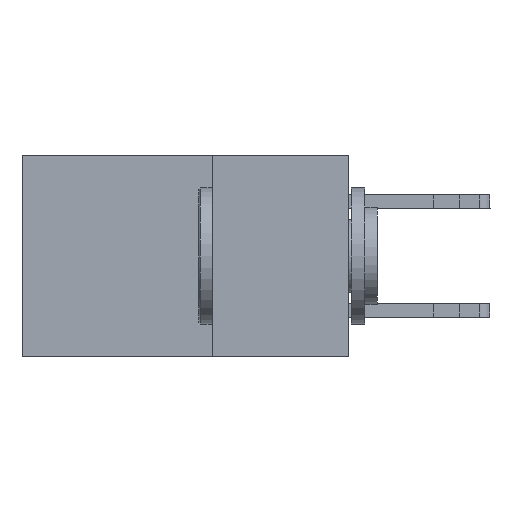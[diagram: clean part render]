
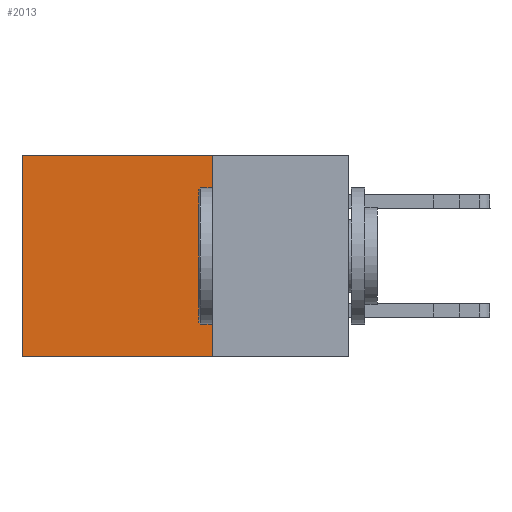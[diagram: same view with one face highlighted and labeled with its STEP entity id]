
A CAD part, left-side view. The second image highlights one B-rep face of the part: STEP entity #2013.
In plain terms, the highlighted planar face has unit normal (-1, 0, 0).
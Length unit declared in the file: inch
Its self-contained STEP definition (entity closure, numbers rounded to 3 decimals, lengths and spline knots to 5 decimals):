
#376 = CARTESIAN_POINT ( 'NONE',  ( 0.2615, 0.25, -0.37 ) ) ;
#753 = EDGE_LOOP ( 'NONE', ( #884, #5151, #13641, #5971 ) ) ;
#847 = CARTESIAN_POINT ( 'NONE',  ( 0.2615, 0.6, -0.37 ) ) ;
#884 = ORIENTED_EDGE ( 'NONE', *, *, #1803, .T. ) ;
#984 = CARTESIAN_POINT ( 'NONE',  ( 0.2615, 0.25, -0.37 ) ) ;
#1065 = FACE_OUTER_BOUND ( 'NONE', #753, .T. ) ;
#1489 = CARTESIAN_POINT ( 'NONE',  ( 0.2615, 0.6, 0. ) ) ;
#1803 = EDGE_CURVE ( 'NONE', #11280, #7477, #9476, .T. ) ;
#2013 = ADVANCED_FACE ( 'NONE', ( #1065 ), #5429, .F. ) ;
#2033 = EDGE_CURVE ( 'NONE', #10538, #4197, #12306, .T. ) ;
#2345 = CARTESIAN_POINT ( 'NONE',  ( 0.2615, 0.25, -0.37 ) ) ;
#3727 = EDGE_CURVE ( 'NONE', #4197, #7477, #8338, .T. ) ;
#4197 = VERTEX_POINT ( 'NONE', #376 ) ;
#4408 = CARTESIAN_POINT ( 'NONE',  ( 0.2615, 0.25, 0. ) ) ;
#5151 = ORIENTED_EDGE ( 'NONE', *, *, #3727, .F. ) ;
#5202 = DIRECTION ( 'NONE',  ( 0., 1., 0. ) ) ;
#5429 = PLANE ( 'NONE',  #5940 ) ;
#5575 = DIRECTION ( 'NONE',  ( 1., 0., 0. ) ) ;
#5940 = AXIS2_PLACEMENT_3D ( 'NONE', #984, #5575, #10065 ) ;
#5971 = ORIENTED_EDGE ( 'NONE', *, *, #13372, .T. ) ;
#6360 = VECTOR ( 'NONE', #7772, 39.37008 ) ;
#7138 = VECTOR ( 'NONE', #13490, 39.37008 ) ;
#7477 = VERTEX_POINT ( 'NONE', #847 ) ;
#7772 = DIRECTION ( 'NONE',  ( 0., 1., 0. ) ) ;
#7912 = VECTOR ( 'NONE', #5202, 39.37008 ) ;
#7992 = LINE ( 'NONE', #4408, #6360 ) ;
#8338 = LINE ( 'NONE', #8638, #7912 ) ;
#8351 = CARTESIAN_POINT ( 'NONE',  ( 0.2615, 0.6, -0.37 ) ) ;
#8638 = CARTESIAN_POINT ( 'NONE',  ( 0.2615, 0.25, -0.37 ) ) ;
#9476 = LINE ( 'NONE', #8351, #12608 ) ;
#10065 = DIRECTION ( 'NONE',  ( 0., 0., -1. ) ) ;
#10538 = VERTEX_POINT ( 'NONE', #14540 ) ;
#11280 = VERTEX_POINT ( 'NONE', #1489 ) ;
#12306 = LINE ( 'NONE', #2345, #7138 ) ;
#12608 = VECTOR ( 'NONE', #12928, 39.37008 ) ;
#12928 = DIRECTION ( 'NONE',  ( 0., 0., -1. ) ) ;
#13372 = EDGE_CURVE ( 'NONE', #10538, #11280, #7992, .T. ) ;
#13490 = DIRECTION ( 'NONE',  ( 0., 0., -1. ) ) ;
#13641 = ORIENTED_EDGE ( 'NONE', *, *, #2033, .F. ) ;
#14540 = CARTESIAN_POINT ( 'NONE',  ( 0.2615, 0.25, 0. ) ) ;
